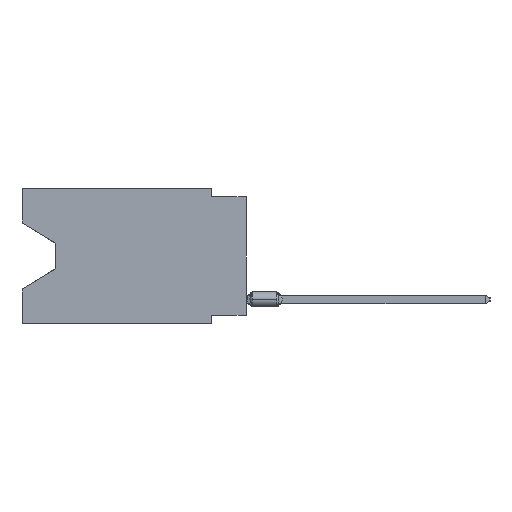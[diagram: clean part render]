
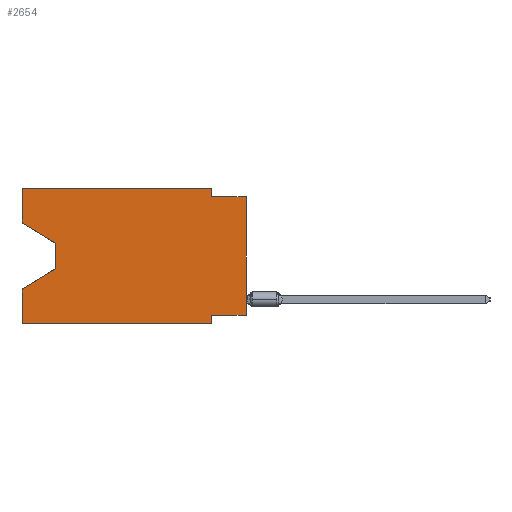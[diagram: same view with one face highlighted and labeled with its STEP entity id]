
A CAD part, left-side view. The second image highlights one B-rep face of the part: STEP entity #2654.
In plain terms, the highlighted planar face has unit normal (-1, 0, 0).
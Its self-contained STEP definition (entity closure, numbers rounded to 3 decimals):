
#386 = DIRECTION ( 'NONE',  ( 0., 0., 1. ) ) ;
#1147 = EDGE_CURVE ( 'NONE', #2702, #28114, #4366, .T. ) ;
#1315 = VECTOR ( 'NONE', #37087, 1000. ) ;
#1598 = DIRECTION ( 'NONE',  ( 0., 0., -1. ) ) ;
#1625 = CARTESIAN_POINT ( 'NONE',  ( 0., 0., 0. ) ) ;
#1709 = ORIENTED_EDGE ( 'NONE', *, *, #1147, .T. ) ;
#2042 = VERTEX_POINT ( 'NONE', #17813 ) ;
#2317 = ORIENTED_EDGE ( 'NONE', *, *, #14131, .F. ) ;
#2457 = ORIENTED_EDGE ( 'NONE', *, *, #16986, .F. ) ;
#2654 = ADVANCED_FACE ( 'NONE', ( #12526 ), #36470, .F. ) ;
#2702 = VERTEX_POINT ( 'NONE', #21760 ) ;
#3181 = LINE ( 'NONE', #15198, #17361 ) ;
#3279 = EDGE_CURVE ( 'NONE', #17610, #17492, #33188, .T. ) ;
#3449 = CARTESIAN_POINT ( 'NONE',  ( 0., 16.383, 0. ) ) ;
#3488 = LINE ( 'NONE', #10163, #1315 ) ;
#3543 = CARTESIAN_POINT ( 'NONE',  ( 0., 0., -0.635 ) ) ;
#4173 = DIRECTION ( 'NONE',  ( 0., 0., 1. ) ) ;
#4330 = EDGE_CURVE ( 'NONE', #2042, #21540, #38437, .T. ) ;
#4366 = LINE ( 'NONE', #1625, #11826 ) ;
#5080 = ORIENTED_EDGE ( 'NONE', *, *, #37028, .F. ) ;
#6502 = LINE ( 'NONE', #25014, #32363 ) ;
#6503 = ORIENTED_EDGE ( 'NONE', *, *, #8741, .F. ) ;
#8158 = CARTESIAN_POINT ( 'NONE',  ( 0., 13.97, -5.893 ) ) ;
#8741 = EDGE_CURVE ( 'NONE', #2702, #31648, #11486, .T. ) ;
#8802 = VERTEX_POINT ( 'NONE', #29724 ) ;
#9483 = CARTESIAN_POINT ( 'NONE',  ( 0., 16.383, 0. ) ) ;
#9591 = CARTESIAN_POINT ( 'NONE',  ( 0., 13.97, -5.893 ) ) ;
#9917 = ORIENTED_EDGE ( 'NONE', *, *, #33953, .T. ) ;
#10163 = CARTESIAN_POINT ( 'NONE',  ( 0., 16.383, 0. ) ) ;
#10452 = CARTESIAN_POINT ( 'NONE',  ( 0., 2.54, -9.906 ) ) ;
#10754 = ORIENTED_EDGE ( 'NONE', *, *, #24480, .F. ) ;
#11486 = LINE ( 'NONE', #32498, #32227 ) ;
#11753 = DIRECTION ( 'NONE',  ( 0., -1., 0. ) ) ;
#11806 = LINE ( 'NONE', #18465, #28129 ) ;
#11826 = VECTOR ( 'NONE', #4173, 1000. ) ;
#11994 = DIRECTION ( 'NONE',  ( 0., 0.855, -0.519 ) ) ;
#12461 = CARTESIAN_POINT ( 'NONE',  ( 0., 2.54, -0.635 ) ) ;
#12526 = FACE_OUTER_BOUND ( 'NONE', #15014, .T. ) ;
#13868 = ORIENTED_EDGE ( 'NONE', *, *, #21586, .T. ) ;
#14131 = EDGE_CURVE ( 'NONE', #2042, #17492, #11806, .T. ) ;
#15014 = EDGE_LOOP ( 'NONE', ( #13868, #9917, #17024, #2317, #23265, #19778, #6503, #1709, #5080, #18766, #2457, #10754 ) ) ;
#15081 = CARTESIAN_POINT ( 'NONE',  ( 0., 13.97, -4.013 ) ) ;
#15198 = CARTESIAN_POINT ( 'NONE',  ( 0., 16.383, 0. ) ) ;
#15279 = CARTESIAN_POINT ( 'NONE',  ( 0., 16.383, -9.906 ) ) ;
#15542 = CARTESIAN_POINT ( 'NONE',  ( 0., 16.383, -7.36 ) ) ;
#16050 = DIRECTION ( 'NONE',  ( 0., 0., -1. ) ) ;
#16556 = LINE ( 'NONE', #10452, #36970 ) ;
#16563 = CARTESIAN_POINT ( 'NONE',  ( 0., 2.54, -9.271 ) ) ;
#16662 = CARTESIAN_POINT ( 'NONE',  ( 0., 2.54, 0. ) ) ;
#16986 = EDGE_CURVE ( 'NONE', #22276, #28452, #3181, .T. ) ;
#17024 = ORIENTED_EDGE ( 'NONE', *, *, #3279, .T. ) ;
#17361 = VECTOR ( 'NONE', #38538, 1000. ) ;
#17492 = VERTEX_POINT ( 'NONE', #15542 ) ;
#17610 = VERTEX_POINT ( 'NONE', #8158 ) ;
#17813 = CARTESIAN_POINT ( 'NONE',  ( 0., 16.383, -9.906 ) ) ;
#18347 = VECTOR ( 'NONE', #27045, 1000. ) ;
#18465 = CARTESIAN_POINT ( 'NONE',  ( 0., 16.383, 0. ) ) ;
#18766 = ORIENTED_EDGE ( 'NONE', *, *, #24462, .F. ) ;
#18849 = DIRECTION ( 'NONE',  ( 0., 0., -1. ) ) ;
#19778 = ORIENTED_EDGE ( 'NONE', *, *, #28891, .F. ) ;
#21091 = CARTESIAN_POINT ( 'NONE',  ( 0., 13.97, -4.013 ) ) ;
#21540 = VERTEX_POINT ( 'NONE', #30850 ) ;
#21586 = EDGE_CURVE ( 'NONE', #8802, #36919, #6502, .T. ) ;
#21760 = CARTESIAN_POINT ( 'NONE',  ( 0., 0., -9.271 ) ) ;
#22276 = VERTEX_POINT ( 'NONE', #9483 ) ;
#23265 = ORIENTED_EDGE ( 'NONE', *, *, #4330, .T. ) ;
#23395 = VERTEX_POINT ( 'NONE', #12461 ) ;
#24462 = EDGE_CURVE ( 'NONE', #28452, #23395, #30387, .T. ) ;
#24480 = EDGE_CURVE ( 'NONE', #8802, #22276, #3488, .T. ) ;
#24719 = CARTESIAN_POINT ( 'NONE',  ( 0., 2.54, 0. ) ) ;
#25014 = CARTESIAN_POINT ( 'NONE',  ( 0., 16.383, -2.546 ) ) ;
#27045 = DIRECTION ( 'NONE',  ( 0., 0., -1. ) ) ;
#27294 = VECTOR ( 'NONE', #27536, 1000. ) ;
#27536 = DIRECTION ( 'NONE',  ( 0., -1., 0. ) ) ;
#28114 = VERTEX_POINT ( 'NONE', #34719 ) ;
#28129 = VECTOR ( 'NONE', #386, 1000. ) ;
#28452 = VERTEX_POINT ( 'NONE', #16662 ) ;
#28891 = EDGE_CURVE ( 'NONE', #31648, #21540, #16556, .T. ) ;
#29724 = CARTESIAN_POINT ( 'NONE',  ( 0., 16.383, -2.546 ) ) ;
#30154 = LINE ( 'NONE', #15081, #18347 ) ;
#30163 = VECTOR ( 'NONE', #18849, 1000. ) ;
#30387 = LINE ( 'NONE', #24719, #30163 ) ;
#30441 = LINE ( 'NONE', #3543, #27294 ) ;
#30466 = AXIS2_PLACEMENT_3D ( 'NONE', #3449, #30743, #16050 ) ;
#30743 = DIRECTION ( 'NONE',  ( 1., 0., 0. ) ) ;
#30850 = CARTESIAN_POINT ( 'NONE',  ( 0., 2.54, -9.906 ) ) ;
#31648 = VERTEX_POINT ( 'NONE', #16563 ) ;
#32227 = VECTOR ( 'NONE', #38201, 1000. ) ;
#32363 = VECTOR ( 'NONE', #33422, 1000. ) ;
#32498 = CARTESIAN_POINT ( 'NONE',  ( 0., 0., -9.271 ) ) ;
#33006 = VECTOR ( 'NONE', #11994, 1000. ) ;
#33188 = LINE ( 'NONE', #9591, #33006 ) ;
#33422 = DIRECTION ( 'NONE',  ( 0., -0.855, -0.519 ) ) ;
#33953 = EDGE_CURVE ( 'NONE', #36919, #17610, #30154, .T. ) ;
#34719 = CARTESIAN_POINT ( 'NONE',  ( 0., 0., -0.635 ) ) ;
#36470 = PLANE ( 'NONE',  #30466 ) ;
#36758 = VECTOR ( 'NONE', #11753, 1000. ) ;
#36919 = VERTEX_POINT ( 'NONE', #21091 ) ;
#36970 = VECTOR ( 'NONE', #1598, 1000. ) ;
#37028 = EDGE_CURVE ( 'NONE', #23395, #28114, #30441, .T. ) ;
#37087 = DIRECTION ( 'NONE',  ( 0., 0., 1. ) ) ;
#38201 = DIRECTION ( 'NONE',  ( 0., 1., 0. ) ) ;
#38437 = LINE ( 'NONE', #15279, #36758 ) ;
#38538 = DIRECTION ( 'NONE',  ( 0., -1., 0. ) ) ;
